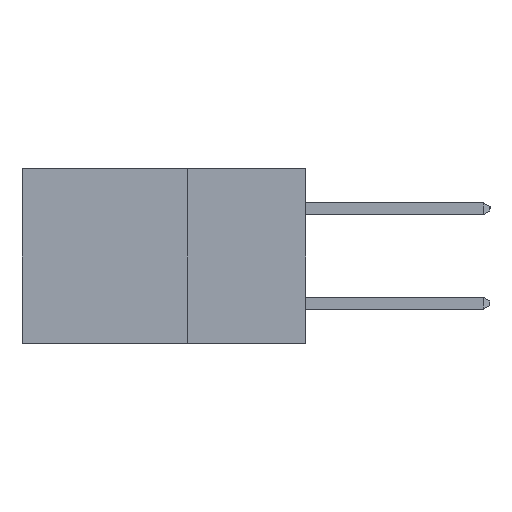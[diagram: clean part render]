
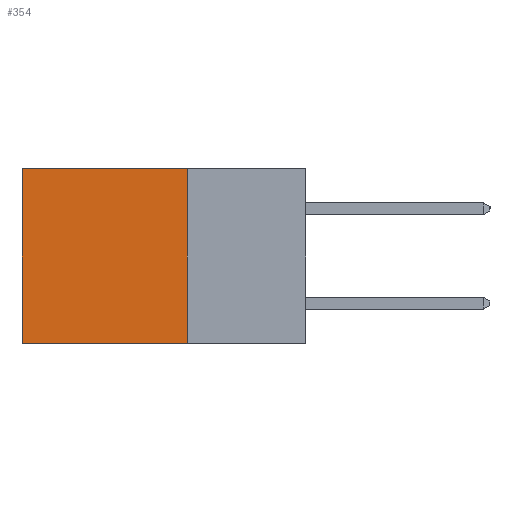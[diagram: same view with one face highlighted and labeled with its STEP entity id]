
A CAD part, left-side view. The second image highlights one B-rep face of the part: STEP entity #354.
In plain terms, the highlighted planar face has unit normal (-1, 0, 0).
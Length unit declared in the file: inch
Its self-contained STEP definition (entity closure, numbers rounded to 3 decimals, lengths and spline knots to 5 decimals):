
#354 = ADVANCED_FACE ( 'NONE', ( #21278 ), #15786, .F. ) ;
#2135 = VECTOR ( 'NONE', #19661, 39.37008 ) ;
#2255 = VECTOR ( 'NONE', #18131, 39.37008 ) ;
#3501 = CARTESIAN_POINT ( 'NONE',  ( 0.2615, 0.6, -0.37 ) ) ;
#4339 = DIRECTION ( 'NONE',  ( 0., 1., 0. ) ) ;
#4453 = LINE ( 'NONE', #5857, #14522 ) ;
#5065 = ORIENTED_EDGE ( 'NONE', *, *, #21110, .F. ) ;
#5664 = VERTEX_POINT ( 'NONE', #19620 ) ;
#5790 = VERTEX_POINT ( 'NONE', #18565 ) ;
#5857 = CARTESIAN_POINT ( 'NONE',  ( 0.2615, 0.25, 0. ) ) ;
#6290 = DIRECTION ( 'NONE',  ( 0., 1., 0. ) ) ;
#6998 = CARTESIAN_POINT ( 'NONE',  ( 0.2615, 0.6, -0.37 ) ) ;
#7078 = DIRECTION ( 'NONE',  ( 1., 0., 0. ) ) ;
#7144 = ORIENTED_EDGE ( 'NONE', *, *, #22835, .T. ) ;
#8594 = DIRECTION ( 'NONE',  ( 0., 0., -1. ) ) ;
#9779 = VERTEX_POINT ( 'NONE', #15746 ) ;
#10229 = ORIENTED_EDGE ( 'NONE', *, *, #12309, .F. ) ;
#11040 = LINE ( 'NONE', #14532, #2255 ) ;
#12119 = ORIENTED_EDGE ( 'NONE', *, *, #13737, .T. ) ;
#12309 = EDGE_CURVE ( 'NONE', #5664, #9779, #11040, .T. ) ;
#13039 = LINE ( 'NONE', #13259, #18401 ) ;
#13259 = CARTESIAN_POINT ( 'NONE',  ( 0.2615, 0.25, -0.37 ) ) ;
#13737 = EDGE_CURVE ( 'NONE', #5664, #5790, #4453, .T. ) ;
#14522 = VECTOR ( 'NONE', #4339, 39.37008 ) ;
#14532 = CARTESIAN_POINT ( 'NONE',  ( 0.2615, 0.25, -0.37 ) ) ;
#14583 = AXIS2_PLACEMENT_3D ( 'NONE', #19283, #7078, #8594 ) ;
#15746 = CARTESIAN_POINT ( 'NONE',  ( 0.2615, 0.25, -0.37 ) ) ;
#15786 = PLANE ( 'NONE',  #14583 ) ;
#16585 = EDGE_LOOP ( 'NONE', ( #7144, #5065, #10229, #12119 ) ) ;
#18131 = DIRECTION ( 'NONE',  ( 0., 0., -1. ) ) ;
#18401 = VECTOR ( 'NONE', #6290, 39.37008 ) ;
#18565 = CARTESIAN_POINT ( 'NONE',  ( 0.2615, 0.6, 0. ) ) ;
#19283 = CARTESIAN_POINT ( 'NONE',  ( 0.2615, 0.25, -0.37 ) ) ;
#19620 = CARTESIAN_POINT ( 'NONE',  ( 0.2615, 0.25, 0. ) ) ;
#19661 = DIRECTION ( 'NONE',  ( 0., 0., -1. ) ) ;
#19816 = VERTEX_POINT ( 'NONE', #6998 ) ;
#21110 = EDGE_CURVE ( 'NONE', #9779, #19816, #13039, .T. ) ;
#21278 = FACE_OUTER_BOUND ( 'NONE', #16585, .T. ) ;
#22705 = LINE ( 'NONE', #3501, #2135 ) ;
#22835 = EDGE_CURVE ( 'NONE', #5790, #19816, #22705, .T. ) ;
